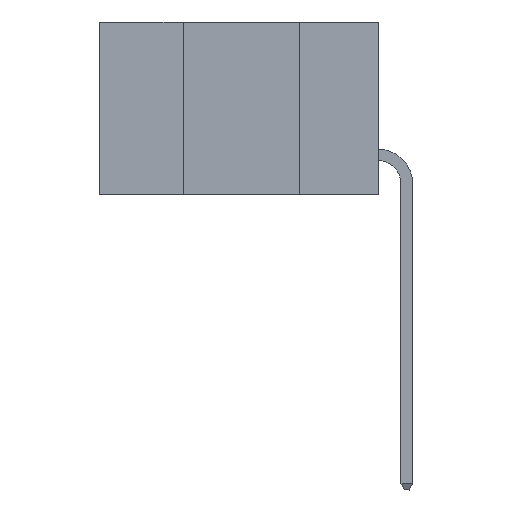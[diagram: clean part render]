
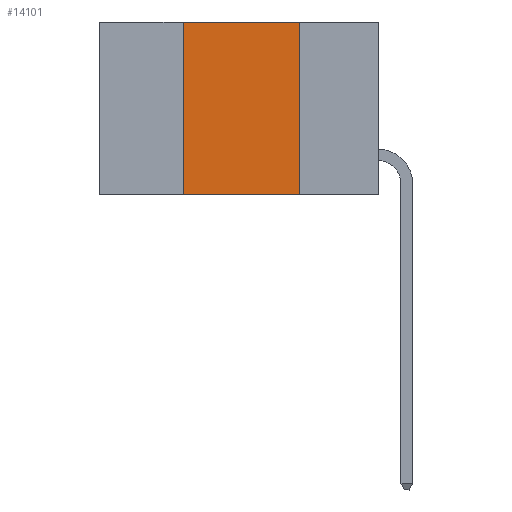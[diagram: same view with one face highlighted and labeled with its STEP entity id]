
A CAD part, left-side view. The second image highlights one B-rep face of the part: STEP entity #14101.
In plain terms, the highlighted planar face has unit normal (-1, 0, 0).
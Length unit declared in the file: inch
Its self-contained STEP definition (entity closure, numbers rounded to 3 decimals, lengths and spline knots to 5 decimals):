
#283 = DIRECTION ( 'NONE',  ( 0., 0., -1. ) ) ;
#376 = VECTOR ( 'NONE', #8768, 39.37008 ) ;
#1263 = LINE ( 'NONE', #20313, #7982 ) ;
#1325 = FACE_OUTER_BOUND ( 'NONE', #18175, .T. ) ;
#1970 = VERTEX_POINT ( 'NONE', #8564 ) ;
#2361 = CARTESIAN_POINT ( 'NONE',  ( 0., 0.42, -0.37 ) ) ;
#2365 = CARTESIAN_POINT ( 'NONE',  ( 0., 0.42, -0.37 ) ) ;
#2579 = ORIENTED_EDGE ( 'NONE', *, *, #12317, .F. ) ;
#2703 = EDGE_CURVE ( 'NONE', #7825, #8374, #3660, .T. ) ;
#3010 = ORIENTED_EDGE ( 'NONE', *, *, #9928, .F. ) ;
#3579 = VERTEX_POINT ( 'NONE', #5422 ) ;
#3660 = LINE ( 'NONE', #14985, #376 ) ;
#5422 = CARTESIAN_POINT ( 'NONE',  ( 0., 0.17, 0. ) ) ;
#6762 = LINE ( 'NONE', #2365, #11645 ) ;
#6848 = CARTESIAN_POINT ( 'NONE',  ( 0., 0.6, 0. ) ) ;
#7155 = DIRECTION ( 'NONE',  ( 0., 0., 1. ) ) ;
#7761 = ORIENTED_EDGE ( 'NONE', *, *, #2703, .T. ) ;
#7825 = VERTEX_POINT ( 'NONE', #2361 ) ;
#7982 = VECTOR ( 'NONE', #15152, 39.37008 ) ;
#8374 = VERTEX_POINT ( 'NONE', #17486 ) ;
#8564 = CARTESIAN_POINT ( 'NONE',  ( 0., 0.42, 0. ) ) ;
#8768 = DIRECTION ( 'NONE',  ( 0., -1., 0. ) ) ;
#9928 = EDGE_CURVE ( 'NONE', #3579, #8374, #1263, .T. ) ;
#10727 = AXIS2_PLACEMENT_3D ( 'NONE', #19087, #14388, #283 ) ;
#11645 = VECTOR ( 'NONE', #7155, 39.37008 ) ;
#12298 = EDGE_CURVE ( 'NONE', #7825, #1970, #6762, .T. ) ;
#12317 = EDGE_CURVE ( 'NONE', #1970, #3579, #17781, .T. ) ;
#14101 = ADVANCED_FACE ( 'NONE', ( #1325 ), #17141, .F. ) ;
#14388 = DIRECTION ( 'NONE',  ( 1., 0., 0. ) ) ;
#14985 = CARTESIAN_POINT ( 'NONE',  ( 0., 0.6, -0.37 ) ) ;
#15152 = DIRECTION ( 'NONE',  ( 0., 0., -1. ) ) ;
#16555 = DIRECTION ( 'NONE',  ( 0., -1., 0. ) ) ;
#17141 = PLANE ( 'NONE',  #10727 ) ;
#17234 = VECTOR ( 'NONE', #16555, 39.37008 ) ;
#17486 = CARTESIAN_POINT ( 'NONE',  ( 0., 0.17, -0.37 ) ) ;
#17781 = LINE ( 'NONE', #6848, #17234 ) ;
#18175 = EDGE_LOOP ( 'NONE', ( #3010, #2579, #18267, #7761 ) ) ;
#18267 = ORIENTED_EDGE ( 'NONE', *, *, #12298, .F. ) ;
#19087 = CARTESIAN_POINT ( 'NONE',  ( 0., 0.6, 0. ) ) ;
#20313 = CARTESIAN_POINT ( 'NONE',  ( 0., 0.17, -0.37 ) ) ;
